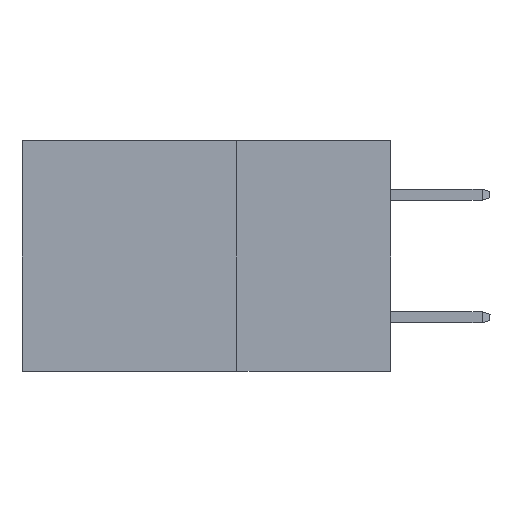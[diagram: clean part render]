
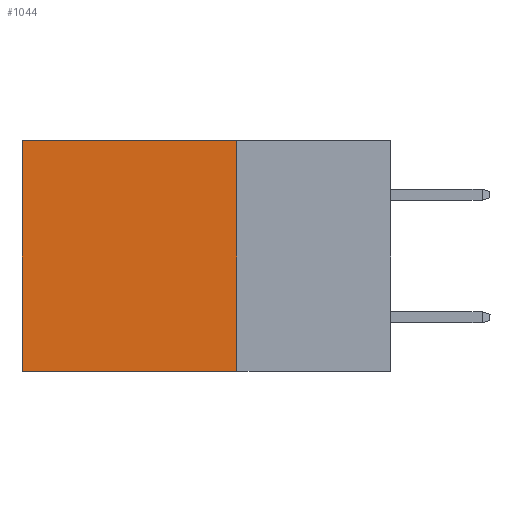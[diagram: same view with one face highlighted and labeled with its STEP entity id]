
A CAD part, left-side view. The second image highlights one B-rep face of the part: STEP entity #1044.
In plain terms, the highlighted planar face has unit normal (-1, 0, 0).
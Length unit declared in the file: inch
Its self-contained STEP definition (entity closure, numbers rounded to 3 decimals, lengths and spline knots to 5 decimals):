
#284 = LINE ( 'NONE', #15910, #16696 ) ;
#641 = CARTESIAN_POINT ( 'NONE',  ( 0.2875, 0.6, 0. ) ) ;
#796 = EDGE_CURVE ( 'NONE', #11946, #7496, #284, .T. ) ;
#996 = VECTOR ( 'NONE', #10740, 39.37008 ) ;
#1044 = ADVANCED_FACE ( 'NONE', ( #5781 ), #10648, .F. ) ;
#1481 = LINE ( 'NONE', #6555, #996 ) ;
#1823 = CARTESIAN_POINT ( 'NONE',  ( 0.2875, 0.25, -0.375 ) ) ;
#2001 = DIRECTION ( 'NONE',  ( 1., 0., 0. ) ) ;
#2137 = DIRECTION ( 'NONE',  ( 0., 0., -1. ) ) ;
#2961 = EDGE_CURVE ( 'NONE', #11946, #3941, #17991, .T. ) ;
#3941 = VERTEX_POINT ( 'NONE', #4685 ) ;
#4685 = CARTESIAN_POINT ( 'NONE',  ( 0.2875, 0.25, -0.375 ) ) ;
#5763 = ORIENTED_EDGE ( 'NONE', *, *, #796, .T. ) ;
#5781 = FACE_OUTER_BOUND ( 'NONE', #10084, .T. ) ;
#6242 = EDGE_CURVE ( 'NONE', #3941, #16681, #1481, .T. ) ;
#6555 = CARTESIAN_POINT ( 'NONE',  ( 0.2875, 0.25, -0.375 ) ) ;
#7496 = VERTEX_POINT ( 'NONE', #641 ) ;
#9005 = CARTESIAN_POINT ( 'NONE',  ( 0.2875, 0.25, -0.375 ) ) ;
#9747 = EDGE_CURVE ( 'NONE', #7496, #16681, #10687, .T. ) ;
#10084 = EDGE_LOOP ( 'NONE', ( #12375, #17345, #15335, #5763 ) ) ;
#10593 = DIRECTION ( 'NONE',  ( 0., 0., -1. ) ) ;
#10648 = PLANE ( 'NONE',  #11621 ) ;
#10687 = LINE ( 'NONE', #10952, #18223 ) ;
#10712 = CARTESIAN_POINT ( 'NONE',  ( 0.2875, 0.25, 0. ) ) ;
#10740 = DIRECTION ( 'NONE',  ( 0., 1., 0. ) ) ;
#10952 = CARTESIAN_POINT ( 'NONE',  ( 0.2875, 0.6, -0.375 ) ) ;
#11621 = AXIS2_PLACEMENT_3D ( 'NONE', #9005, #2001, #12175 ) ;
#11946 = VERTEX_POINT ( 'NONE', #10712 ) ;
#12175 = DIRECTION ( 'NONE',  ( 0., 0., -1. ) ) ;
#12375 = ORIENTED_EDGE ( 'NONE', *, *, #9747, .T. ) ;
#14150 = CARTESIAN_POINT ( 'NONE',  ( 0.2875, 0.6, -0.375 ) ) ;
#15335 = ORIENTED_EDGE ( 'NONE', *, *, #2961, .F. ) ;
#15910 = CARTESIAN_POINT ( 'NONE',  ( 0.2875, 0.25, 0. ) ) ;
#15969 = DIRECTION ( 'NONE',  ( 0., 1., 0. ) ) ;
#16681 = VERTEX_POINT ( 'NONE', #14150 ) ;
#16696 = VECTOR ( 'NONE', #15969, 39.37008 ) ;
#17061 = VECTOR ( 'NONE', #10593, 39.37008 ) ;
#17345 = ORIENTED_EDGE ( 'NONE', *, *, #6242, .F. ) ;
#17991 = LINE ( 'NONE', #1823, #17061 ) ;
#18223 = VECTOR ( 'NONE', #2137, 39.37008 ) ;
